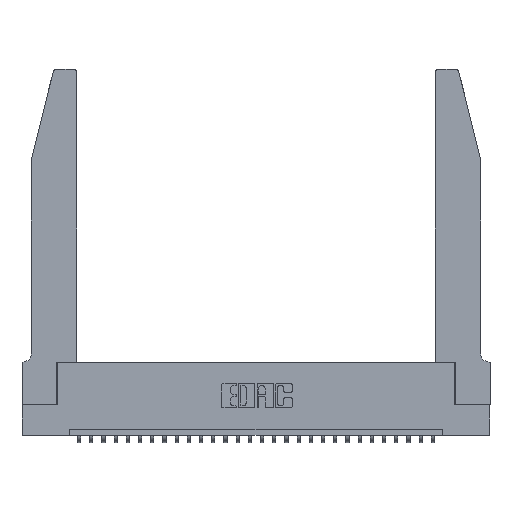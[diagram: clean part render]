
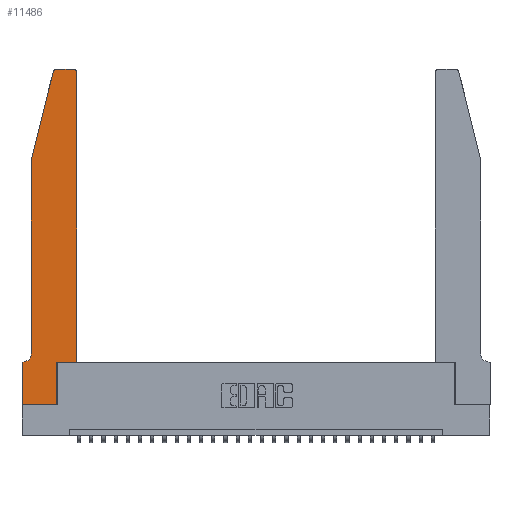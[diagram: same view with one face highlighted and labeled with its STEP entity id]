
A CAD part, top view. The second image highlights one B-rep face of the part: STEP entity #11486.
In plain terms, the highlighted planar face has unit normal (0, 0, 1).
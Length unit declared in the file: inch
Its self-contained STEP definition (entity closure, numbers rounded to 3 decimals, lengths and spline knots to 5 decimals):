
#22 = VECTOR ( 'NONE', #1382, 39.37008 ) ;
#81 = DIRECTION ( 'NONE',  ( 0., 1., 0. ) ) ;
#90 = EDGE_CURVE ( 'NONE', #3368, #14673, #15174, .T. ) ;
#173 = ORIENTED_EDGE ( 'NONE', *, *, #19726, .T. ) ;
#367 = CARTESIAN_POINT ( 'NONE',  ( 0.25487, 2.72718, 0.37 ) ) ;
#418 = VECTOR ( 'NONE', #28091, 39.37008 ) ;
#478 = VECTOR ( 'NONE', #9938, 39.37008 ) ;
#862 = FACE_OUTER_BOUND ( 'NONE', #6444, .T. ) ;
#879 = DIRECTION ( 'NONE',  ( 0., 0., 1. ) ) ;
#1073 = CARTESIAN_POINT ( 'NONE',  ( 0.0755, 2., 0.37 ) ) ;
#1382 = DIRECTION ( 'NONE',  ( 1., 0., 0. ) ) ;
#1783 = AXIS2_PLACEMENT_3D ( 'NONE', #7940, #879, #25455 ) ;
#2047 = VECTOR ( 'NONE', #29045, 39.37008 ) ;
#2141 = CARTESIAN_POINT ( 'NONE',  ( 0., 0., 0.37 ) ) ;
#2172 = CARTESIAN_POINT ( 'NONE',  ( 0., 0.35, 0.37 ) ) ;
#2244 = ORIENTED_EDGE ( 'NONE', *, *, #9603, .T. ) ;
#2422 = DIRECTION ( 'NONE',  ( 0., 1., 0. ) ) ;
#3368 = VERTEX_POINT ( 'NONE', #14470 ) ;
#3635 = VERTEX_POINT ( 'NONE', #2141 ) ;
#3843 = DIRECTION ( 'NONE',  ( -1., 0., 0. ) ) ;
#4575 = LINE ( 'NONE', #13585, #22 ) ;
#4599 = VERTEX_POINT ( 'NONE', #12520 ) ;
#5147 = VERTEX_POINT ( 'NONE', #19624 ) ;
#5148 = CARTESIAN_POINT ( 'NONE',  ( 0.0755, 0.35, 0.37 ) ) ;
#5317 = ORIENTED_EDGE ( 'NONE', *, *, #22334, .T. ) ;
#5406 = DIRECTION ( 'NONE',  ( 1., 0., 0. ) ) ;
#5763 = CARTESIAN_POINT ( 'NONE',  ( 0.2865, 0.35, 0.37 ) ) ;
#6073 = CARTESIAN_POINT ( 'NONE',  ( 0., 0., 0.37 ) ) ;
#6100 = VERTEX_POINT ( 'NONE', #19514 ) ;
#6159 = VECTOR ( 'NONE', #28399, 39.37008 ) ;
#6444 = EDGE_LOOP ( 'NONE', ( #28094, #7252, #18741, #5317, #23604, #14621, #14507, #13592, #12359, #19072, #173, #2244 ) ) ;
#7188 = LINE ( 'NONE', #6073, #6159 ) ;
#7209 = EDGE_CURVE ( 'NONE', #6100, #28910, #17162, .T. ) ;
#7252 = ORIENTED_EDGE ( 'NONE', *, *, #22282, .T. ) ;
#7504 = VECTOR ( 'NONE', #3843, 39.37008 ) ;
#7940 = CARTESIAN_POINT ( 'NONE',  ( 0.284, 2.72, 0.37 ) ) ;
#8913 = LINE ( 'NONE', #5148, #7504 ) ;
#9278 = LINE ( 'NONE', #27159, #26440 ) ;
#9603 = EDGE_CURVE ( 'NONE', #26056, #27638, #16344, .T. ) ;
#9816 = CARTESIAN_POINT ( 'NONE',  ( 0.4505, 2.72, 0.37 ) ) ;
#9938 = DIRECTION ( 'NONE',  ( -0.239, -0.971, 0. ) ) ;
#10025 = DIRECTION ( 'NONE',  ( 0., 0., -1. ) ) ;
#10140 = LINE ( 'NONE', #22114, #2047 ) ;
#10662 = CARTESIAN_POINT ( 'NONE',  ( 0.0755, 2., 0.37 ) ) ;
#11191 = VECTOR ( 'NONE', #81, 39.37008 ) ;
#11486 = ADVANCED_FACE ( 'NONE', ( #862 ), #13349, .T. ) ;
#11574 = DIRECTION ( 'NONE',  ( 0., 0., 1. ) ) ;
#11799 = CARTESIAN_POINT ( 'NONE',  ( 0.4205, 2.75, 0.37 ) ) ;
#11857 = AXIS2_PLACEMENT_3D ( 'NONE', #2172, #11574, #27251 ) ;
#12359 = ORIENTED_EDGE ( 'NONE', *, *, #7209, .T. ) ;
#12520 = CARTESIAN_POINT ( 'NONE',  ( 0.4505, 0.35, 0.37 ) ) ;
#12921 = EDGE_CURVE ( 'NONE', #3635, #6100, #4575, .T. ) ;
#13349 = PLANE ( 'NONE',  #11857 ) ;
#13585 = CARTESIAN_POINT ( 'NONE',  ( 0., 0., 0.37 ) ) ;
#13592 = ORIENTED_EDGE ( 'NONE', *, *, #12921, .T. ) ;
#14271 = CARTESIAN_POINT ( 'NONE',  ( 0.0055, 0.35, 0.37 ) ) ;
#14300 = EDGE_CURVE ( 'NONE', #28910, #4599, #10140, .T. ) ;
#14470 = CARTESIAN_POINT ( 'NONE',  ( 0.0755, 0.42, 0.37 ) ) ;
#14507 = ORIENTED_EDGE ( 'NONE', *, *, #20233, .T. ) ;
#14621 = ORIENTED_EDGE ( 'NONE', *, *, #20769, .T. ) ;
#14673 = VERTEX_POINT ( 'NONE', #14271 ) ;
#14850 = LINE ( 'NONE', #1073, #418 ) ;
#15174 = CIRCLE ( 'NONE', #25927, 0.07 ) ;
#15615 = VERTEX_POINT ( 'NONE', #367 ) ;
#15777 = LINE ( 'NONE', #18904, #20647 ) ;
#16344 = CIRCLE ( 'NONE', #28161, 0.03 ) ;
#17162 = LINE ( 'NONE', #17554, #11191 ) ;
#17554 = CARTESIAN_POINT ( 'NONE',  ( 0.2865, 0.35, 0.37 ) ) ;
#18055 = DIRECTION ( 'NONE',  ( -1., 0., 0. ) ) ;
#18575 = VERTEX_POINT ( 'NONE', #10662 ) ;
#18741 = ORIENTED_EDGE ( 'NONE', *, *, #21429, .T. ) ;
#18904 = CARTESIAN_POINT ( 'NONE',  ( 0.4505, 0.35, 0.37 ) ) ;
#18921 = CARTESIAN_POINT ( 'NONE',  ( 0.0055, 0.42, 0.37 ) ) ;
#19072 = ORIENTED_EDGE ( 'NONE', *, *, #14300, .T. ) ;
#19514 = CARTESIAN_POINT ( 'NONE',  ( 0.2865, 0., 0.37 ) ) ;
#19611 = DIRECTION ( 'NONE',  ( -1., 0., 0. ) ) ;
#19624 = CARTESIAN_POINT ( 'NONE',  ( 0., 0.35, 0.37 ) ) ;
#19726 = EDGE_CURVE ( 'NONE', #4599, #26056, #15777, .T. ) ;
#20233 = EDGE_CURVE ( 'NONE', #5147, #3635, #7188, .T. ) ;
#20474 = EDGE_CURVE ( 'NONE', #27638, #28313, #9278, .T. ) ;
#20647 = VECTOR ( 'NONE', #2422, 39.37008 ) ;
#20769 = EDGE_CURVE ( 'NONE', #14673, #5147, #8913, .T. ) ;
#21173 = CARTESIAN_POINT ( 'NONE',  ( 0.284, 2.75, 0.37 ) ) ;
#21429 = EDGE_CURVE ( 'NONE', #15615, #18575, #27471, .T. ) ;
#22114 = CARTESIAN_POINT ( 'NONE',  ( 0.4505, 0.35, 0.37 ) ) ;
#22282 = EDGE_CURVE ( 'NONE', #28313, #15615, #28836, .T. ) ;
#22334 = EDGE_CURVE ( 'NONE', #18575, #3368, #14850, .T. ) ;
#23604 = ORIENTED_EDGE ( 'NONE', *, *, #90, .T. ) ;
#25455 = DIRECTION ( 'NONE',  ( 1., 0., 0. ) ) ;
#25474 = CARTESIAN_POINT ( 'NONE',  ( 0.4205, 2.72, 0.37 ) ) ;
#25687 = CARTESIAN_POINT ( 'NONE',  ( 0.0755, 2., 0.37 ) ) ;
#25927 = AXIS2_PLACEMENT_3D ( 'NONE', #18921, #10025, #19611 ) ;
#26056 = VERTEX_POINT ( 'NONE', #9816 ) ;
#26167 = DIRECTION ( 'NONE',  ( 0., 0., 1. ) ) ;
#26440 = VECTOR ( 'NONE', #18055, 39.37008 ) ;
#27159 = CARTESIAN_POINT ( 'NONE',  ( 0.2605, 2.75, 0.37 ) ) ;
#27251 = DIRECTION ( 'NONE',  ( 1., 0., 0. ) ) ;
#27471 = LINE ( 'NONE', #25687, #478 ) ;
#27638 = VERTEX_POINT ( 'NONE', #11799 ) ;
#28091 = DIRECTION ( 'NONE',  ( 0., -1., 0. ) ) ;
#28094 = ORIENTED_EDGE ( 'NONE', *, *, #20474, .T. ) ;
#28161 = AXIS2_PLACEMENT_3D ( 'NONE', #25474, #26167, #5406 ) ;
#28313 = VERTEX_POINT ( 'NONE', #21173 ) ;
#28399 = DIRECTION ( 'NONE',  ( 0., -1., 0. ) ) ;
#28836 = CIRCLE ( 'NONE', #1783, 0.03 ) ;
#28910 = VERTEX_POINT ( 'NONE', #5763 ) ;
#29045 = DIRECTION ( 'NONE',  ( 1., 0., 0. ) ) ;
